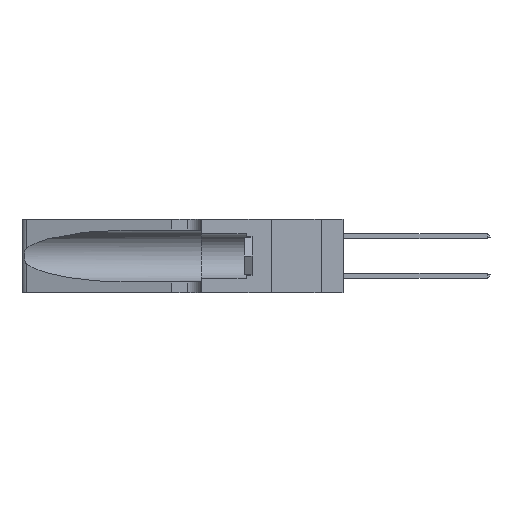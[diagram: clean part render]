
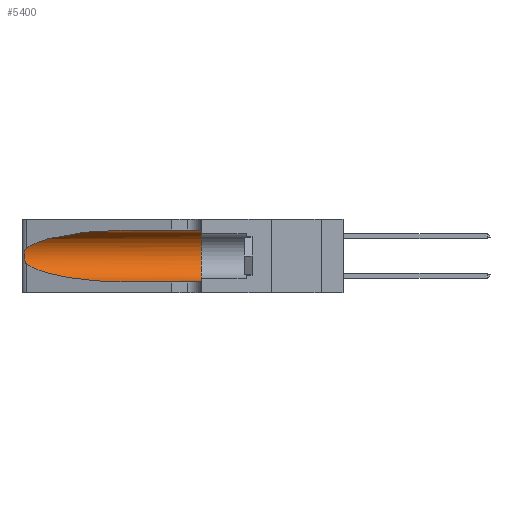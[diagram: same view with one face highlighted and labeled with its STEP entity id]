
A CAD part, left-side view. The second image highlights one B-rep face of the part: STEP entity #5400.
In plain terms, the highlighted cylindrical face has radius 3.308 mm (diameter 6.617 mm), a partial arc.
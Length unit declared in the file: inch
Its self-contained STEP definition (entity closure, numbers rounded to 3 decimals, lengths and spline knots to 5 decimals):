
#1029 = CARTESIAN_POINT ( 'NONE',  ( 0.1305, 1.61858, 0.05475 ) ) ;
#1355 = AXIS2_PLACEMENT_3D ( 'NONE', #23054, #17824, #6912 ) ;
#1993 = B_SPLINE_CURVE_WITH_KNOTS ( 'NONE', 3,
 ( #10589, #12359, #14169, #3157, #15962, #5053, #17769, #6941, #19551, #8807, #21299, #10662, #23082, #12441 ),
 .UNSPECIFIED., .F., .F.,
 ( 4, 2, 2, 2, 2, 2, 4 ),
 ( 0., 0.00027, 0.00053, 0.00107, 0.0016, 0.00187, 0.00214 ),
 .UNSPECIFIED. ) ;
#2536 = VERTEX_POINT ( 'NONE', #5453 ) ;
#2942 = VECTOR ( 'NONE', #8588, 39.37008 ) ;
#3157 = CARTESIAN_POINT ( 'NONE',  ( 0.25787, 1.23484, 0.2124 ) ) ;
#3263 = CARTESIAN_POINT ( 'NONE',  ( 0.1305, 0.35, 0.185 ) ) ;
#3467 = CARTESIAN_POINT ( 'NONE',  ( 0.1305, 0.72297, 0.31525 ) ) ;
#4479 = CARTESIAN_POINT ( 'NONE',  ( 0.1305, 1.61858, 0.31525 ) ) ;
#4658 = CARTESIAN_POINT ( 'NONE',  ( 0.25487, 1.22718, 0.14631 ) ) ;
#4970 = CARTESIAN_POINT ( 'NONE',  ( 0.18966, 0.96281, 0.31525 ) ) ;
#5010 = CYLINDRICAL_SURFACE ( 'NONE', #1355, 0.13025 ) ;
#5053 = CARTESIAN_POINT ( 'NONE',  ( 0.26018, 1.23835, 0.19895 ) ) ;
#5173 = DIRECTION ( 'NONE',  ( 0., 0., 1. ) ) ;
#5400 = ADVANCED_FACE ( 'NONE', ( #15301 ), #5010, .F. ) ;
#5453 = CARTESIAN_POINT ( 'NONE',  ( 0.1305, 0.72297, 0.05475 ) ) ;
#5919 = EDGE_CURVE ( 'NONE', #21475, #2536, #23048, .T. ) ;
#5976 = EDGE_CURVE ( 'NONE', #2536, #15168, #12783, .T. ) ;
#5997 = ORIENTED_EDGE ( 'NONE', *, *, #11810, .T. ) ;
#6209 = CIRCLE ( 'NONE', #8098, 0.13025 ) ;
#6412 = VECTOR ( 'NONE', #19036, 39.37008 ) ;
#6769 = EDGE_CURVE ( 'NONE', #14629, #17962, #18987, .T. ) ;
#6912 = DIRECTION ( 'NONE',  ( 0., 0., -1. ) ) ;
#6941 = CARTESIAN_POINT ( 'NONE',  ( 0.26075, 1.23896, 0.178 ) ) ;
#8098 = AXIS2_PLACEMENT_3D ( 'NONE', #3263, #16070, #5173 ) ;
#8428 = CARTESIAN_POINT ( 'NONE',  ( 0.18966, 0.96281, 0.05475 ) ) ;
#8588 = DIRECTION ( 'NONE',  ( 0., -1., 0. ) ) ;
#8807 = CARTESIAN_POINT ( 'NONE',  ( 0.25856, 1.23593, 0.16098 ) ) ;
#9691 = EDGE_CURVE ( 'NONE', #14629, #18807, #11858, .T. ) ;
#10498 = CARTESIAN_POINT ( 'NONE',  ( 0.1305, 0.72297, 0.31525 ) ) ;
#10589 = CARTESIAN_POINT ( 'NONE',  ( 0.25487, 1.22718, 0.22369 ) ) ;
#10662 = CARTESIAN_POINT ( 'NONE',  ( 0.25639, 1.23186, 0.15144 ) ) ;
#10845 = ORIENTED_EDGE ( 'NONE', *, *, #5919, .T. ) ;
#11810 = EDGE_CURVE ( 'NONE', #17962, #21475, #1993, .T. ) ;
#11858 = LINE ( 'NONE', #4479, #6412 ) ;
#12346 = ORIENTED_EDGE ( 'NONE', *, *, #16246, .F. ) ;
#12359 = CARTESIAN_POINT ( 'NONE',  ( 0.25555, 1.22994, 0.2215 ) ) ;
#12441 = CARTESIAN_POINT ( 'NONE',  ( 0.25487, 1.22718, 0.14631 ) ) ;
#12783 = LINE ( 'NONE', #1029, #2942 ) ;
#13053 = ORIENTED_EDGE ( 'NONE', *, *, #5976, .T. ) ;
#13589 = ORIENTED_EDGE ( 'NONE', *, *, #9691, .F. ) ;
#13957 = CARTESIAN_POINT ( 'NONE',  ( 0.25487, 1.22718, 0.22369 ) ) ;
#14169 = CARTESIAN_POINT ( 'NONE',  ( 0.25639, 1.23184, 0.21858 ) ) ;
#14629 = VERTEX_POINT ( 'NONE', #3467 ) ;
#15168 = VERTEX_POINT ( 'NONE', #19663 ) ;
#15301 = FACE_OUTER_BOUND ( 'NONE', #17060, .T. ) ;
#15346 = CARTESIAN_POINT ( 'NONE',  ( 0.25487, 1.22718, 0.14631 ) ) ;
#15605 = CARTESIAN_POINT ( 'NONE',  ( 0.2373, 1.15595, 0.08982 ) ) ;
#15884 = CARTESIAN_POINT ( 'NONE',  ( 0.2373, 1.15595, 0.28018 ) ) ;
#15962 = CARTESIAN_POINT ( 'NONE',  ( 0.25854, 1.2359, 0.20912 ) ) ;
#16070 = DIRECTION ( 'NONE',  ( 0., 1., 0. ) ) ;
#16246 = EDGE_CURVE ( 'NONE', #18807, #15168, #6209, .T. ) ;
#16391 = CARTESIAN_POINT ( 'NONE',  ( 0.1305, 0.35, 0.31525 ) ) ;
#17060 = EDGE_LOOP ( 'NONE', ( #23202, #5997, #10845, #13053, #12346, #13589 ) ) ;
#17693 = CARTESIAN_POINT ( 'NONE',  ( 0.25487, 1.22718, 0.22369 ) ) ;
#17769 = CARTESIAN_POINT ( 'NONE',  ( 0.26075, 1.23896, 0.19203 ) ) ;
#17824 = DIRECTION ( 'NONE',  ( 0., -1., 0. ) ) ;
#17962 = VERTEX_POINT ( 'NONE', #13957 ) ;
#18807 = VERTEX_POINT ( 'NONE', #16391 ) ;
#18987 =( BOUNDED_CURVE ( )  B_SPLINE_CURVE ( 3, ( #10498, #4970, #15884, #17693 ),
 .UNSPECIFIED., .F., .F. ) 
 B_SPLINE_CURVE_WITH_KNOTS ( ( 4, 4 ),
 ( 1.5708, 2.84003 ),
 .UNSPECIFIED. ) 
 CURVE ( )  GEOMETRIC_REPRESENTATION_ITEM ( )  RATIONAL_B_SPLINE_CURVE ( ( 1., 0.87, 0.87, 1. ) ) 
 REPRESENTATION_ITEM ( '' )  );
#19036 = DIRECTION ( 'NONE',  ( 0., -1., 0. ) ) ;
#19551 = CARTESIAN_POINT ( 'NONE',  ( 0.26017, 1.23833, 0.17102 ) ) ;
#19663 = CARTESIAN_POINT ( 'NONE',  ( 0.1305, 0.35, 0.05475 ) ) ;
#20946 = CARTESIAN_POINT ( 'NONE',  ( 0.1305, 0.72297, 0.05475 ) ) ;
#21299 = CARTESIAN_POINT ( 'NONE',  ( 0.25789, 1.23486, 0.15765 ) ) ;
#21475 = VERTEX_POINT ( 'NONE', #15346 ) ;
#23048 =( BOUNDED_CURVE ( )  B_SPLINE_CURVE ( 3, ( #4658, #15605, #8428, #20946 ),
 .UNSPECIFIED., .F., .F. ) 
 B_SPLINE_CURVE_WITH_KNOTS ( ( 4, 4 ),
 ( 3.44316, 4.71239 ),
 .UNSPECIFIED. ) 
 CURVE ( )  GEOMETRIC_REPRESENTATION_ITEM ( )  RATIONAL_B_SPLINE_CURVE ( ( 1., 0.87, 0.87, 1. ) ) 
 REPRESENTATION_ITEM ( '' )  );
#23054 = CARTESIAN_POINT ( 'NONE',  ( 0.1305, 1.61858, 0.185 ) ) ;
#23082 = CARTESIAN_POINT ( 'NONE',  ( 0.25555, 1.22993, 0.14849 ) ) ;
#23202 = ORIENTED_EDGE ( 'NONE', *, *, #6769, .T. ) ;
